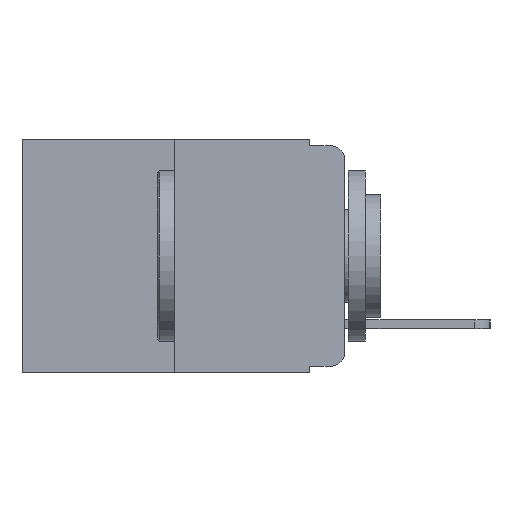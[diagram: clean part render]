
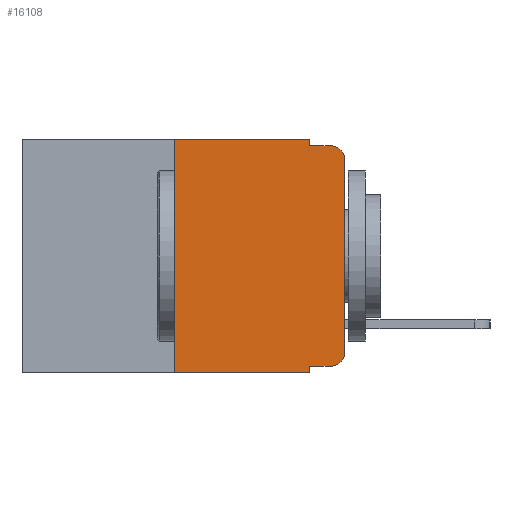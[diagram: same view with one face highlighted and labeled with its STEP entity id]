
A CAD part, left-side view. The second image highlights one B-rep face of the part: STEP entity #16108.
In plain terms, the highlighted planar face has unit normal (-1, 0, 0).
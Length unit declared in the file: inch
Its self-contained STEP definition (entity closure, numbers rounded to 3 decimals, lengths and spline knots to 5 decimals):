
#7 = EDGE_CURVE ( 'NONE', #2556, #12226, #9486, .T. ) ;
#46 = EDGE_CURVE ( 'NONE', #12226, #3155, #12277, .T. ) ;
#54 = EDGE_CURVE ( 'NONE', #13812, #3155, #7889, .T. ) ;
#90 = EDGE_CURVE ( 'NONE', #17782, #13812, #7368, .T. ) ;
#94 = EDGE_CURVE ( 'NONE', #16349, #8760, #10751, .T. ) ;
#119 = EDGE_CURVE ( 'NONE', #9606, #13343, #9740, .T. ) ;
#128 = EDGE_CURVE ( 'NONE', #9606, #12433, #13548, .T. ) ;
#161 = EDGE_CURVE ( 'NONE', #12433, #2556, #16929, .T. ) ;
#477 = DIRECTION ( 'NONE',  ( 0., 0., 1. ) ) ;
#1052 = CARTESIAN_POINT ( 'NONE',  ( 0., 0.02, -0.03 ) ) ;
#1711 = DIRECTION ( 'NONE',  ( 0., 0., 1. ) ) ;
#1782 = DIRECTION ( 'NONE',  ( -1., 0., 0. ) ) ;
#2372 = CARTESIAN_POINT ( 'NONE',  ( 0., 0., 0. ) ) ;
#2520 = CARTESIAN_POINT ( 'NONE',  ( 0., 0.25, 0. ) ) ;
#2535 = CARTESIAN_POINT ( 'NONE',  ( 0., 0.051, -0.333 ) ) ;
#2556 = VERTEX_POINT ( 'NONE', #15172 ) ;
#2611 = CARTESIAN_POINT ( 'NONE',  ( 0., 0.051, 0. ) ) ;
#2711 = DIRECTION ( 'NONE',  ( 0., 0., -1. ) ) ;
#2738 = CARTESIAN_POINT ( 'NONE',  ( 0., 0.051, 0. ) ) ;
#2961 = CARTESIAN_POINT ( 'NONE',  ( 0., 0.02, -0.333 ) ) ;
#2987 = EDGE_CURVE ( 'NONE', #8760, #17782, #6337, .T. ) ;
#3155 = VERTEX_POINT ( 'NONE', #20165 ) ;
#3221 = DIRECTION ( 'NONE',  ( 0., -1., 0. ) ) ;
#3548 = CARTESIAN_POINT ( 'NONE',  ( 0., 0.051, -0.343 ) ) ;
#3857 = CARTESIAN_POINT ( 'NONE',  ( 0., 0.02, -0.313 ) ) ;
#4271 = VECTOR ( 'NONE', #1711, 39.37008 ) ;
#4542 = VECTOR ( 'NONE', #13809, 39.37008 ) ;
#5023 = ORIENTED_EDGE ( 'NONE', *, *, #161, .T. ) ;
#5297 = ORIENTED_EDGE ( 'NONE', *, *, #90, .F. ) ;
#6337 = LINE ( 'NONE', #11404, #21699 ) ;
#6804 = DIRECTION ( 'NONE',  ( 1., 0., 0. ) ) ;
#7025 = DIRECTION ( 'NONE',  ( 0., -1., 0. ) ) ;
#7368 = LINE ( 'NONE', #2738, #18911 ) ;
#7533 = ORIENTED_EDGE ( 'NONE', *, *, #94, .F. ) ;
#7889 = LINE ( 'NONE', #20070, #11765 ) ;
#8608 = ORIENTED_EDGE ( 'NONE', *, *, #119, .F. ) ;
#8760 = VERTEX_POINT ( 'NONE', #13670 ) ;
#9383 = ORIENTED_EDGE ( 'NONE', *, *, #46, .T. ) ;
#9486 = LINE ( 'NONE', #2372, #4271 ) ;
#9606 = VERTEX_POINT ( 'NONE', #2535 ) ;
#9740 = LINE ( 'NONE', #2611, #17912 ) ;
#9998 = LINE ( 'NONE', #15296, #17676 ) ;
#10248 = VECTOR ( 'NONE', #477, 39.37008 ) ;
#10751 = LINE ( 'NONE', #2520, #10248 ) ;
#11404 = CARTESIAN_POINT ( 'NONE',  ( 0., 0.473, 0. ) ) ;
#11691 = EDGE_LOOP ( 'NONE', ( #16571, #9383, #18066, #5297, #20085, #7533, #21078, #8608, #13463, #5023 ) ) ;
#11765 = VECTOR ( 'NONE', #3221, 39.37008 ) ;
#12226 = VERTEX_POINT ( 'NONE', #16208 ) ;
#12249 = CARTESIAN_POINT ( 'NONE',  ( 0., 0.25, -0.343 ) ) ;
#12277 = CIRCLE ( 'NONE', #22107, 0.02 ) ;
#12433 = VERTEX_POINT ( 'NONE', #2961 ) ;
#13122 = AXIS2_PLACEMENT_3D ( 'NONE', #19883, #6804, #18355 ) ;
#13343 = VERTEX_POINT ( 'NONE', #3548 ) ;
#13463 = ORIENTED_EDGE ( 'NONE', *, *, #128, .T. ) ;
#13548 = LINE ( 'NONE', #13789, #4542 ) ;
#13670 = CARTESIAN_POINT ( 'NONE',  ( 0., 0.25, 0. ) ) ;
#13789 = CARTESIAN_POINT ( 'NONE',  ( 0., 0.051, -0.333 ) ) ;
#13809 = DIRECTION ( 'NONE',  ( 0., -1., 0. ) ) ;
#13812 = VERTEX_POINT ( 'NONE', #16319 ) ;
#14188 = EDGE_CURVE ( 'NONE', #16349, #13343, #9998, .T. ) ;
#15172 = CARTESIAN_POINT ( 'NONE',  ( 0., 0., -0.313 ) ) ;
#15296 = CARTESIAN_POINT ( 'NONE',  ( 0., 0.473, -0.343 ) ) ;
#16108 = ADVANCED_FACE ( 'NONE', ( #21871 ), #16751, .F. ) ;
#16208 = CARTESIAN_POINT ( 'NONE',  ( 0., 0., -0.03 ) ) ;
#16319 = CARTESIAN_POINT ( 'NONE',  ( 0., 0.051, -0.01 ) ) ;
#16349 = VERTEX_POINT ( 'NONE', #12249 ) ;
#16571 = ORIENTED_EDGE ( 'NONE', *, *, #7, .T. ) ;
#16751 = PLANE ( 'NONE',  #13122 ) ;
#16929 = CIRCLE ( 'NONE', #21745, 0.02 ) ;
#17676 = VECTOR ( 'NONE', #7025, 39.37008 ) ;
#17782 = VERTEX_POINT ( 'NONE', #21655 ) ;
#17912 = VECTOR ( 'NONE', #18797, 39.37008 ) ;
#18066 = ORIENTED_EDGE ( 'NONE', *, *, #54, .F. ) ;
#18355 = DIRECTION ( 'NONE',  ( 0., 0., -1. ) ) ;
#18797 = DIRECTION ( 'NONE',  ( 0., 0., -1. ) ) ;
#18837 = DIRECTION ( 'NONE',  ( 0., 0., -1. ) ) ;
#18911 = VECTOR ( 'NONE', #2711, 39.37008 ) ;
#19533 = DIRECTION ( 'NONE',  ( 0., -1., 0. ) ) ;
#19883 = CARTESIAN_POINT ( 'NONE',  ( 0., 0.473, 0. ) ) ;
#20070 = CARTESIAN_POINT ( 'NONE',  ( 0., 0.051, -0.01 ) ) ;
#20085 = ORIENTED_EDGE ( 'NONE', *, *, #2987, .F. ) ;
#20088 = DIRECTION ( 'NONE',  ( 0., 0., -1. ) ) ;
#20165 = CARTESIAN_POINT ( 'NONE',  ( 0., 0.02, -0.01 ) ) ;
#20874 = DIRECTION ( 'NONE',  ( -1., 0., 0. ) ) ;
#21078 = ORIENTED_EDGE ( 'NONE', *, *, #14188, .T. ) ;
#21655 = CARTESIAN_POINT ( 'NONE',  ( 0., 0.051, 0. ) ) ;
#21699 = VECTOR ( 'NONE', #19533, 39.37008 ) ;
#21745 = AXIS2_PLACEMENT_3D ( 'NONE', #3857, #1782, #18837 ) ;
#21871 = FACE_OUTER_BOUND ( 'NONE', #11691, .T. ) ;
#22107 = AXIS2_PLACEMENT_3D ( 'NONE', #1052, #20874, #20088 ) ;
